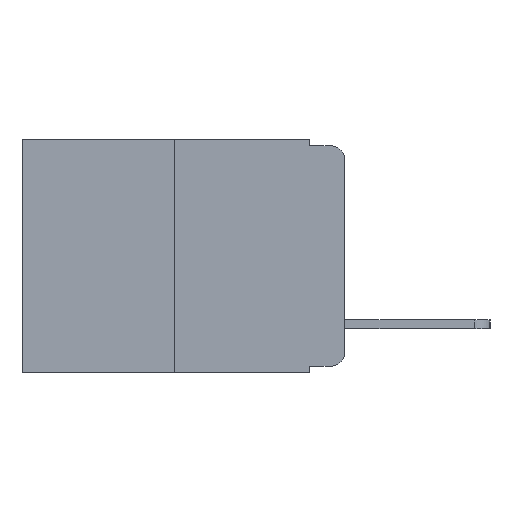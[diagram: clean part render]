
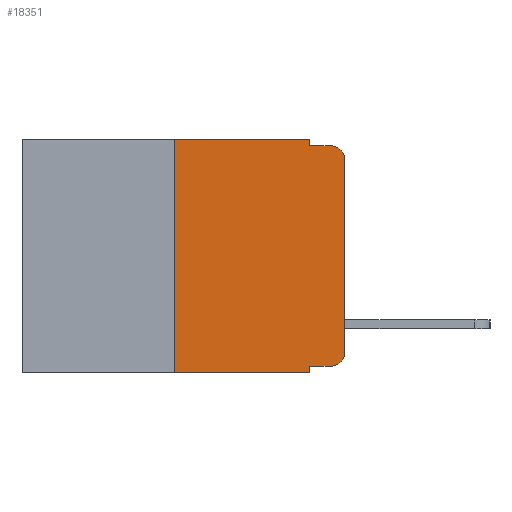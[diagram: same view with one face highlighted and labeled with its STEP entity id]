
A CAD part, left-side view. The second image highlights one B-rep face of the part: STEP entity #18351.
In plain terms, the highlighted planar face has unit normal (-1, 0, 0).
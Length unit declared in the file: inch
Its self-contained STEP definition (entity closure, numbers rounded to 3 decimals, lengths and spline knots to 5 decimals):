
#504 = AXIS2_PLACEMENT_3D ( 'NONE', #687, #12612, #2518 ) ;
#594 = LINE ( 'NONE', #20625, #17674 ) ;
#641 = CARTESIAN_POINT ( 'NONE',  ( 0., 0.051, -0.343 ) ) ;
#687 = CARTESIAN_POINT ( 'NONE',  ( 0., 0.02, -0.313 ) ) ;
#966 = CIRCLE ( 'NONE', #504, 0.02 ) ;
#1135 = EDGE_CURVE ( 'NONE', #19372, #3408, #7489, .T. ) ;
#1291 = VECTOR ( 'NONE', #7795, 39.37008 ) ;
#1509 = CARTESIAN_POINT ( 'NONE',  ( 0., 0.25, 0. ) ) ;
#1516 = CARTESIAN_POINT ( 'NONE',  ( 0., 0., -0.03 ) ) ;
#1783 = DIRECTION ( 'NONE',  ( 0., -1., 0. ) ) ;
#2280 = VERTEX_POINT ( 'NONE', #11606 ) ;
#2513 = ORIENTED_EDGE ( 'NONE', *, *, #3561, .T. ) ;
#2518 = DIRECTION ( 'NONE',  ( 0., 0., -1. ) ) ;
#3171 = AXIS2_PLACEMENT_3D ( 'NONE', #12214, #15363, #5651 ) ;
#3408 = VERTEX_POINT ( 'NONE', #6375 ) ;
#3541 = VECTOR ( 'NONE', #8392, 39.37008 ) ;
#3561 = EDGE_CURVE ( 'NONE', #2280, #17291, #19689, .T. ) ;
#4231 = CARTESIAN_POINT ( 'NONE',  ( 0., 0.051, -0.01 ) ) ;
#4438 = ORIENTED_EDGE ( 'NONE', *, *, #7062, .T. ) ;
#4560 = VERTEX_POINT ( 'NONE', #1516 ) ;
#4793 = LINE ( 'NONE', #18969, #16228 ) ;
#5149 = VERTEX_POINT ( 'NONE', #9033 ) ;
#5651 = DIRECTION ( 'NONE',  ( 0., 0., -1. ) ) ;
#5941 = VERTEX_POINT ( 'NONE', #13233 ) ;
#5957 = CARTESIAN_POINT ( 'NONE',  ( 0., 0.473, 0. ) ) ;
#6375 = CARTESIAN_POINT ( 'NONE',  ( 0., 0.02, -0.01 ) ) ;
#6600 = DIRECTION ( 'NONE',  ( 0., 0., 1. ) ) ;
#6960 = EDGE_CURVE ( 'NONE', #17285, #8318, #18649, .T. ) ;
#7062 = EDGE_CURVE ( 'NONE', #4560, #3408, #19349, .T. ) ;
#7179 = ORIENTED_EDGE ( 'NONE', *, *, #13930, .F. ) ;
#7368 = VECTOR ( 'NONE', #17893, 39.37008 ) ;
#7461 = EDGE_CURVE ( 'NONE', #5149, #11461, #966, .T. ) ;
#7489 = LINE ( 'NONE', #11332, #15501 ) ;
#7635 = FACE_OUTER_BOUND ( 'NONE', #16339, .T. ) ;
#7711 = ORIENTED_EDGE ( 'NONE', *, *, #7461, .T. ) ;
#7795 = DIRECTION ( 'NONE',  ( 0., -1., 0. ) ) ;
#8048 = DIRECTION ( 'NONE',  ( 0., 0., -1. ) ) ;
#8150 = LINE ( 'NONE', #8324, #3541 ) ;
#8318 = VERTEX_POINT ( 'NONE', #18054 ) ;
#8324 = CARTESIAN_POINT ( 'NONE',  ( 0., 0.051, 0. ) ) ;
#8392 = DIRECTION ( 'NONE',  ( 0., 0., -1. ) ) ;
#9027 = ORIENTED_EDGE ( 'NONE', *, *, #1135, .F. ) ;
#9033 = CARTESIAN_POINT ( 'NONE',  ( 0., 0.02, -0.333 ) ) ;
#9227 = CARTESIAN_POINT ( 'NONE',  ( 0., 0., -0.313 ) ) ;
#9863 = CARTESIAN_POINT ( 'NONE',  ( 0., 0.02, -0.03 ) ) ;
#11332 = CARTESIAN_POINT ( 'NONE',  ( 0., 0.051, -0.01 ) ) ;
#11438 = DIRECTION ( 'NONE',  ( 0., 0., -1. ) ) ;
#11461 = VERTEX_POINT ( 'NONE', #9227 ) ;
#11526 = DIRECTION ( 'NONE',  ( 0., -1., 0. ) ) ;
#11548 = LINE ( 'NONE', #16137, #12027 ) ;
#11557 = ORIENTED_EDGE ( 'NONE', *, *, #11867, .T. ) ;
#11606 = CARTESIAN_POINT ( 'NONE',  ( 0., 0.25, -0.343 ) ) ;
#11726 = AXIS2_PLACEMENT_3D ( 'NONE', #9863, #20534, #11438 ) ;
#11741 = LINE ( 'NONE', #1509, #7368 ) ;
#11867 = EDGE_CURVE ( 'NONE', #5941, #5149, #594, .T. ) ;
#12027 = VECTOR ( 'NONE', #6600, 39.37008 ) ;
#12214 = CARTESIAN_POINT ( 'NONE',  ( 0., 0.473, 0. ) ) ;
#12612 = DIRECTION ( 'NONE',  ( -1., 0., 0. ) ) ;
#12753 = CARTESIAN_POINT ( 'NONE',  ( 0., 0.473, -0.343 ) ) ;
#13129 = DIRECTION ( 'NONE',  ( 0., -1., 0. ) ) ;
#13233 = CARTESIAN_POINT ( 'NONE',  ( 0., 0.051, -0.333 ) ) ;
#13728 = ORIENTED_EDGE ( 'NONE', *, *, #20025, .F. ) ;
#13930 = EDGE_CURVE ( 'NONE', #5941, #17291, #4793, .T. ) ;
#14735 = ORIENTED_EDGE ( 'NONE', *, *, #6960, .F. ) ;
#15363 = DIRECTION ( 'NONE',  ( 1., 0., 0. ) ) ;
#15501 = VECTOR ( 'NONE', #1783, 39.37008 ) ;
#15706 = VECTOR ( 'NONE', #13129, 39.37008 ) ;
#15897 = EDGE_CURVE ( 'NONE', #11461, #4560, #11548, .T. ) ;
#16137 = CARTESIAN_POINT ( 'NONE',  ( 0., 0., 0. ) ) ;
#16228 = VECTOR ( 'NONE', #8048, 39.37008 ) ;
#16339 = EDGE_LOOP ( 'NONE', ( #16851, #4438, #9027, #13728, #14735, #18739, #2513, #7179, #11557, #7711 ) ) ;
#16851 = ORIENTED_EDGE ( 'NONE', *, *, #15897, .T. ) ;
#17285 = VERTEX_POINT ( 'NONE', #20119 ) ;
#17291 = VERTEX_POINT ( 'NONE', #641 ) ;
#17674 = VECTOR ( 'NONE', #11526, 39.37008 ) ;
#17893 = DIRECTION ( 'NONE',  ( 0., 0., 1. ) ) ;
#18025 = EDGE_CURVE ( 'NONE', #2280, #17285, #11741, .T. ) ;
#18054 = CARTESIAN_POINT ( 'NONE',  ( 0., 0.051, 0. ) ) ;
#18351 = ADVANCED_FACE ( 'NONE', ( #7635 ), #19821, .F. ) ;
#18649 = LINE ( 'NONE', #5957, #1291 ) ;
#18739 = ORIENTED_EDGE ( 'NONE', *, *, #18025, .F. ) ;
#18969 = CARTESIAN_POINT ( 'NONE',  ( 0., 0.051, 0. ) ) ;
#19349 = CIRCLE ( 'NONE', #11726, 0.02 ) ;
#19372 = VERTEX_POINT ( 'NONE', #4231 ) ;
#19689 = LINE ( 'NONE', #12753, #15706 ) ;
#19821 = PLANE ( 'NONE',  #3171 ) ;
#20025 = EDGE_CURVE ( 'NONE', #8318, #19372, #8150, .T. ) ;
#20119 = CARTESIAN_POINT ( 'NONE',  ( 0., 0.25, 0. ) ) ;
#20534 = DIRECTION ( 'NONE',  ( -1., 0., 0. ) ) ;
#20625 = CARTESIAN_POINT ( 'NONE',  ( 0., 0.051, -0.333 ) ) ;
